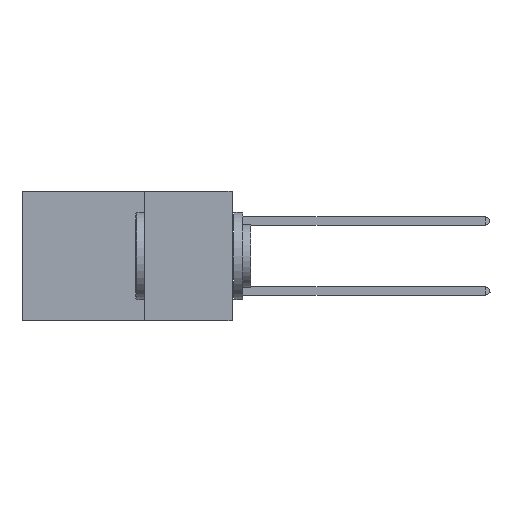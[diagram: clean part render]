
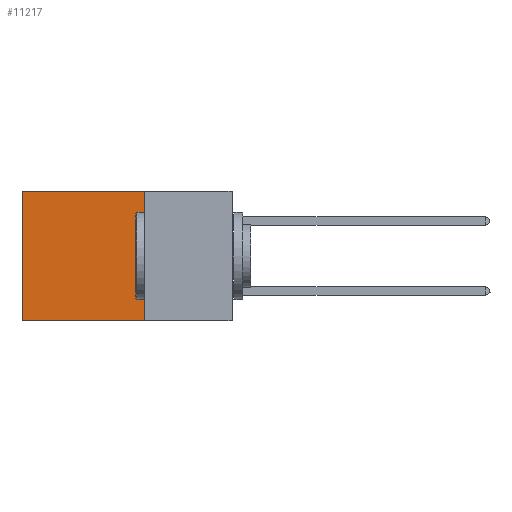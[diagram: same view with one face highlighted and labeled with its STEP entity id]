
A CAD part, left-side view. The second image highlights one B-rep face of the part: STEP entity #11217.
In plain terms, the highlighted planar face has unit normal (-1, 0, 0).
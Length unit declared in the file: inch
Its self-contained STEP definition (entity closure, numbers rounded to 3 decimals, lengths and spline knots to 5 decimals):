
#1204 = VERTEX_POINT ( 'NONE', #25989 ) ;
#2909 = EDGE_CURVE ( 'NONE', #13939, #3931, #24588, .T. ) ;
#3931 = VERTEX_POINT ( 'NONE', #8879 ) ;
#4350 = ORIENTED_EDGE ( 'NONE', *, *, #8598, .F. ) ;
#5661 = LINE ( 'NONE', #14483, #26443 ) ;
#7341 = CARTESIAN_POINT ( 'NONE',  ( 0.2875, 0.25, 0. ) ) ;
#7458 = VECTOR ( 'NONE', #26879, 39.37008 ) ;
#8380 = LINE ( 'NONE', #10709, #16937 ) ;
#8598 = EDGE_CURVE ( 'NONE', #13939, #14159, #8380, .T. ) ;
#8879 = CARTESIAN_POINT ( 'NONE',  ( 0.2875, 0.6, 0. ) ) ;
#10021 = EDGE_LOOP ( 'NONE', ( #20980, #11979, #4350, #12559 ) ) ;
#10709 = CARTESIAN_POINT ( 'NONE',  ( 0.2875, 0.25, 0. ) ) ;
#11217 = ADVANCED_FACE ( 'NONE', ( #13972 ), #13527, .F. ) ;
#11979 = ORIENTED_EDGE ( 'NONE', *, *, #16480, .F. ) ;
#12559 = ORIENTED_EDGE ( 'NONE', *, *, #2909, .T. ) ;
#12802 = LINE ( 'NONE', #20393, #7458 ) ;
#13527 = PLANE ( 'NONE',  #24977 ) ;
#13939 = VERTEX_POINT ( 'NONE', #7341 ) ;
#13972 = FACE_OUTER_BOUND ( 'NONE', #10021, .T. ) ;
#14159 = VERTEX_POINT ( 'NONE', #21607 ) ;
#14483 = CARTESIAN_POINT ( 'NONE',  ( 0.2875, 0.25, -0.37 ) ) ;
#16480 = EDGE_CURVE ( 'NONE', #14159, #1204, #5661, .T. ) ;
#16937 = VECTOR ( 'NONE', #21795, 39.37008 ) ;
#17971 = CARTESIAN_POINT ( 'NONE',  ( 0.2875, 0.25, 0. ) ) ;
#20393 = CARTESIAN_POINT ( 'NONE',  ( 0.2875, 0.6, 0. ) ) ;
#20892 = EDGE_CURVE ( 'NONE', #3931, #1204, #12802, .T. ) ;
#20980 = ORIENTED_EDGE ( 'NONE', *, *, #20892, .T. ) ;
#21607 = CARTESIAN_POINT ( 'NONE',  ( 0.2875, 0.25, -0.37 ) ) ;
#21795 = DIRECTION ( 'NONE',  ( 0., 0., -1. ) ) ;
#22735 = DIRECTION ( 'NONE',  ( 0., 0., -1. ) ) ;
#22833 = DIRECTION ( 'NONE',  ( 1., 0., 0. ) ) ;
#23501 = VECTOR ( 'NONE', #26649, 39.37008 ) ;
#24588 = LINE ( 'NONE', #17971, #23501 ) ;
#24977 = AXIS2_PLACEMENT_3D ( 'NONE', #27188, #22833, #22735 ) ;
#25989 = CARTESIAN_POINT ( 'NONE',  ( 0.2875, 0.6, -0.37 ) ) ;
#26443 = VECTOR ( 'NONE', #28557, 39.37008 ) ;
#26649 = DIRECTION ( 'NONE',  ( 0., 1., 0. ) ) ;
#26879 = DIRECTION ( 'NONE',  ( 0., 0., -1. ) ) ;
#27188 = CARTESIAN_POINT ( 'NONE',  ( 0.2875, 0.25, 0. ) ) ;
#28557 = DIRECTION ( 'NONE',  ( 0., 1., 0. ) ) ;
